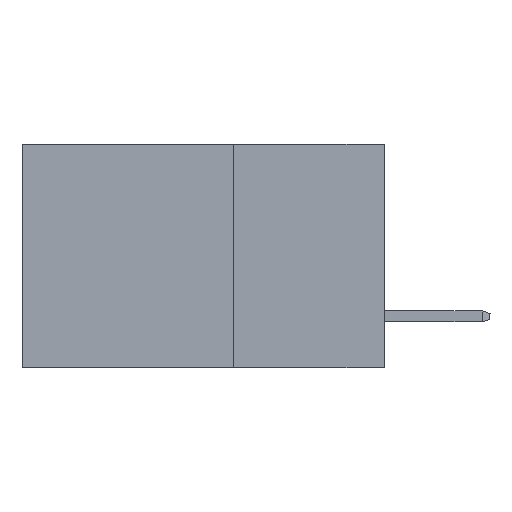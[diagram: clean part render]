
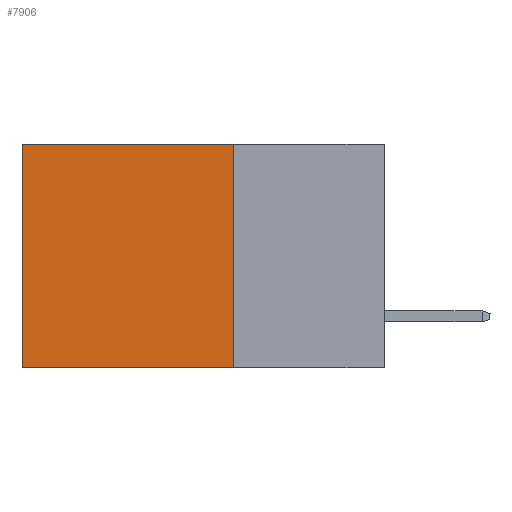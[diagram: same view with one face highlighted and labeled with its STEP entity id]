
A CAD part, left-side view. The second image highlights one B-rep face of the part: STEP entity #7906.
In plain terms, the highlighted planar face has unit normal (-1, 0, 0).
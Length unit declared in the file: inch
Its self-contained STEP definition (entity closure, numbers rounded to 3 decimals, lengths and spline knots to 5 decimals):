
#2435 = VECTOR ( 'NONE', #3267, 39.37008 ) ;
#2501 = AXIS2_PLACEMENT_3D ( 'NONE', #21322, #25431, #19334 ) ;
#2568 = VECTOR ( 'NONE', #23672, 39.37008 ) ;
#2613 = CARTESIAN_POINT ( 'NONE',  ( 0.2615, 0.6, 0. ) ) ;
#2874 = CARTESIAN_POINT ( 'NONE',  ( 0.2615, 0.25, -0.37 ) ) ;
#2886 = VERTEX_POINT ( 'NONE', #26086 ) ;
#3267 = DIRECTION ( 'NONE',  ( 0., 0., -1. ) ) ;
#3298 = CARTESIAN_POINT ( 'NONE',  ( 0.2615, 0.6, -0.37 ) ) ;
#4281 = VECTOR ( 'NONE', #10890, 39.37008 ) ;
#6154 = EDGE_CURVE ( 'NONE', #2886, #13168, #9260, .T. ) ;
#6764 = LINE ( 'NONE', #14745, #4281 ) ;
#6973 = PLANE ( 'NONE',  #2501 ) ;
#7906 = ADVANCED_FACE ( 'NONE', ( #17338 ), #6973, .F. ) ;
#8346 = ORIENTED_EDGE ( 'NONE', *, *, #9835, .F. ) ;
#9073 = ORIENTED_EDGE ( 'NONE', *, *, #21337, .T. ) ;
#9260 = LINE ( 'NONE', #2874, #2435 ) ;
#9835 = EDGE_CURVE ( 'NONE', #13168, #20901, #15595, .T. ) ;
#10890 = DIRECTION ( 'NONE',  ( 0., 1., 0. ) ) ;
#13082 = EDGE_LOOP ( 'NONE', ( #9073, #8346, #15791, #21536 ) ) ;
#13168 = VERTEX_POINT ( 'NONE', #18506 ) ;
#14745 = CARTESIAN_POINT ( 'NONE',  ( 0.2615, 0.25, 0. ) ) ;
#15595 = LINE ( 'NONE', #19959, #2568 ) ;
#15708 = CARTESIAN_POINT ( 'NONE',  ( 0.2615, 0.6, -0.37 ) ) ;
#15791 = ORIENTED_EDGE ( 'NONE', *, *, #6154, .F. ) ;
#17338 = FACE_OUTER_BOUND ( 'NONE', #13082, .T. ) ;
#17660 = DIRECTION ( 'NONE',  ( 0., 0., -1. ) ) ;
#17854 = VECTOR ( 'NONE', #17660, 39.37008 ) ;
#18506 = CARTESIAN_POINT ( 'NONE',  ( 0.2615, 0.25, -0.37 ) ) ;
#19334 = DIRECTION ( 'NONE',  ( 0., 0., -1. ) ) ;
#19959 = CARTESIAN_POINT ( 'NONE',  ( 0.2615, 0.25, -0.37 ) ) ;
#20901 = VERTEX_POINT ( 'NONE', #15708 ) ;
#21125 = EDGE_CURVE ( 'NONE', #2886, #22784, #6764, .T. ) ;
#21322 = CARTESIAN_POINT ( 'NONE',  ( 0.2615, 0.25, -0.37 ) ) ;
#21337 = EDGE_CURVE ( 'NONE', #22784, #20901, #23224, .T. ) ;
#21536 = ORIENTED_EDGE ( 'NONE', *, *, #21125, .T. ) ;
#22784 = VERTEX_POINT ( 'NONE', #2613 ) ;
#23224 = LINE ( 'NONE', #3298, #17854 ) ;
#23672 = DIRECTION ( 'NONE',  ( 0., 1., 0. ) ) ;
#25431 = DIRECTION ( 'NONE',  ( 1., 0., 0. ) ) ;
#26086 = CARTESIAN_POINT ( 'NONE',  ( 0.2615, 0.25, 0. ) ) ;
